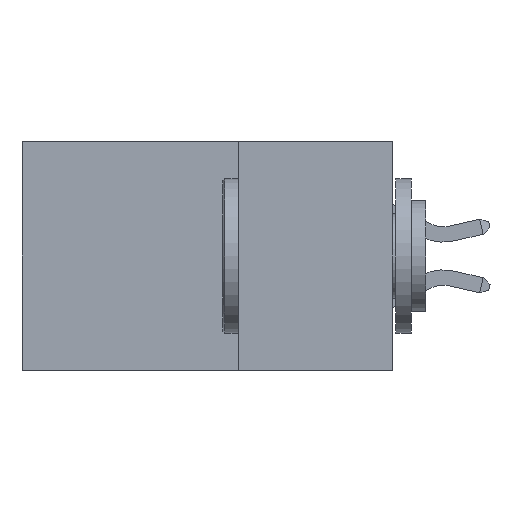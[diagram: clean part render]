
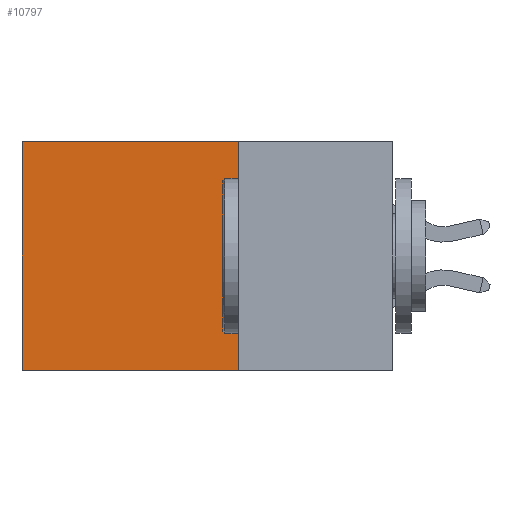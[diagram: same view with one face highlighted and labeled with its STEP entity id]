
A CAD part, left-side view. The second image highlights one B-rep face of the part: STEP entity #10797.
In plain terms, the highlighted planar face has unit normal (-1, 0, 0).
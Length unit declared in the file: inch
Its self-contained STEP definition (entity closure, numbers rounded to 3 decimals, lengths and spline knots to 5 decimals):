
#246 = VERTEX_POINT ( 'NONE', #10694 ) ;
#273 = DIRECTION ( 'NONE',  ( 1., 0., 0. ) ) ;
#494 = AXIS2_PLACEMENT_3D ( 'NONE', #13474, #273, #10805 ) ;
#1636 = LINE ( 'NONE', #6144, #12822 ) ;
#1891 = ORIENTED_EDGE ( 'NONE', *, *, #7889, .T. ) ;
#2523 = DIRECTION ( 'NONE',  ( 0., 1., 0. ) ) ;
#4577 = CARTESIAN_POINT ( 'NONE',  ( 0.2875, 0.25, 0. ) ) ;
#6144 = CARTESIAN_POINT ( 'NONE',  ( 0.2875, 0.6, 0. ) ) ;
#7002 = LINE ( 'NONE', #14858, #10371 ) ;
#7350 = CARTESIAN_POINT ( 'NONE',  ( 0.2875, 0.25, 0. ) ) ;
#7889 = EDGE_CURVE ( 'NONE', #8772, #17805, #11769, .T. ) ;
#7911 = PLANE ( 'NONE',  #494 ) ;
#8024 = EDGE_CURVE ( 'NONE', #17805, #10592, #1636, .T. ) ;
#8321 = VECTOR ( 'NONE', #2523, 39.37008 ) ;
#8772 = VERTEX_POINT ( 'NONE', #4577 ) ;
#8814 = DIRECTION ( 'NONE',  ( 0., 1., 0. ) ) ;
#8948 = EDGE_CURVE ( 'NONE', #8772, #246, #7002, .T. ) ;
#9314 = ORIENTED_EDGE ( 'NONE', *, *, #9772, .F. ) ;
#9772 = EDGE_CURVE ( 'NONE', #246, #10592, #12128, .T. ) ;
#9808 = CARTESIAN_POINT ( 'NONE',  ( 0.2875, 0.25, -0.37 ) ) ;
#10371 = VECTOR ( 'NONE', #16226, 39.37008 ) ;
#10592 = VERTEX_POINT ( 'NONE', #15944 ) ;
#10694 = CARTESIAN_POINT ( 'NONE',  ( 0.2875, 0.25, -0.37 ) ) ;
#10797 = ADVANCED_FACE ( 'NONE', ( #11204 ), #7911, .F. ) ;
#10805 = DIRECTION ( 'NONE',  ( 0., 0., -1. ) ) ;
#11204 = FACE_OUTER_BOUND ( 'NONE', #15055, .T. ) ;
#11769 = LINE ( 'NONE', #7350, #18706 ) ;
#12123 = CARTESIAN_POINT ( 'NONE',  ( 0.2875, 0.6, 0. ) ) ;
#12128 = LINE ( 'NONE', #9808, #8321 ) ;
#12822 = VECTOR ( 'NONE', #17409, 39.37008 ) ;
#13047 = ORIENTED_EDGE ( 'NONE', *, *, #8948, .F. ) ;
#13474 = CARTESIAN_POINT ( 'NONE',  ( 0.2875, 0.25, 0. ) ) ;
#14858 = CARTESIAN_POINT ( 'NONE',  ( 0.2875, 0.25, 0. ) ) ;
#15055 = EDGE_LOOP ( 'NONE', ( #16272, #9314, #13047, #1891 ) ) ;
#15944 = CARTESIAN_POINT ( 'NONE',  ( 0.2875, 0.6, -0.37 ) ) ;
#16226 = DIRECTION ( 'NONE',  ( 0., 0., -1. ) ) ;
#16272 = ORIENTED_EDGE ( 'NONE', *, *, #8024, .T. ) ;
#17409 = DIRECTION ( 'NONE',  ( 0., 0., -1. ) ) ;
#17805 = VERTEX_POINT ( 'NONE', #12123 ) ;
#18706 = VECTOR ( 'NONE', #8814, 39.37008 ) ;
